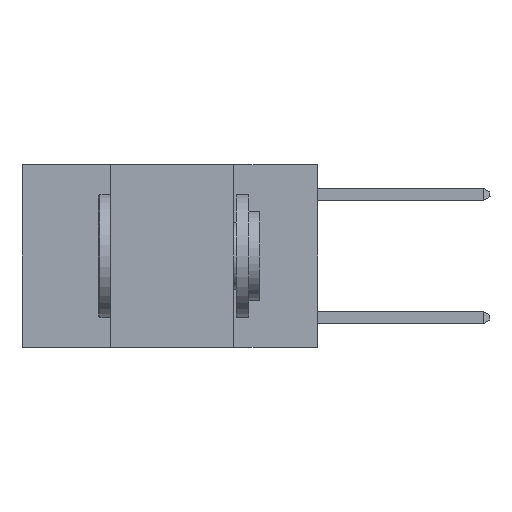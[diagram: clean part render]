
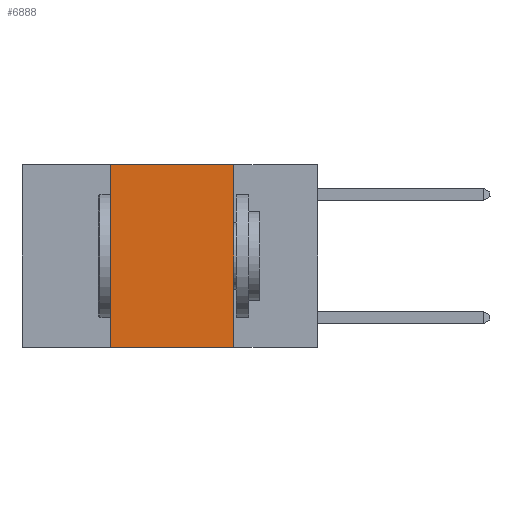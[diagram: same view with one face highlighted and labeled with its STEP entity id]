
A CAD part, left-side view. The second image highlights one B-rep face of the part: STEP entity #6888.
In plain terms, the highlighted planar face has unit normal (-1, 0, 0).
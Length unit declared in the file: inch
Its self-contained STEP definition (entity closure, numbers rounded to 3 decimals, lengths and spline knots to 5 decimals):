
#2115 = DIRECTION ( 'NONE',  ( 0., 0., 1. ) ) ;
#2191 = DIRECTION ( 'NONE',  ( 1., 0., 0. ) ) ;
#2390 = VERTEX_POINT ( 'NONE', #15531 ) ;
#2639 = VECTOR ( 'NONE', #3451, 39.37008 ) ;
#2764 = VECTOR ( 'NONE', #2115, 39.37008 ) ;
#2792 = ORIENTED_EDGE ( 'NONE', *, *, #17667, .F. ) ;
#3072 = CARTESIAN_POINT ( 'NONE',  ( 0., 0.6, 0. ) ) ;
#3198 = EDGE_CURVE ( 'NONE', #15660, #10734, #3631, .T. ) ;
#3207 = VECTOR ( 'NONE', #6868, 39.37008 ) ;
#3451 = DIRECTION ( 'NONE',  ( 0., -1., 0. ) ) ;
#3631 = LINE ( 'NONE', #4788, #10253 ) ;
#4340 = VERTEX_POINT ( 'NONE', #17554 ) ;
#4788 = CARTESIAN_POINT ( 'NONE',  ( 0., 0.17, 0. ) ) ;
#4964 = CARTESIAN_POINT ( 'NONE',  ( 0., 0.6, -0.37 ) ) ;
#6868 = DIRECTION ( 'NONE',  ( 0., -1., 0. ) ) ;
#6888 = ADVANCED_FACE ( 'NONE', ( #14616 ), #8845, .F. ) ;
#7405 = CARTESIAN_POINT ( 'NONE',  ( 0., 0.17, -0.37 ) ) ;
#8462 = LINE ( 'NONE', #3072, #3207 ) ;
#8845 = PLANE ( 'NONE',  #12199 ) ;
#9971 = ORIENTED_EDGE ( 'NONE', *, *, #10574, .T. ) ;
#10092 = CARTESIAN_POINT ( 'NONE',  ( 0., 0.17, 0. ) ) ;
#10253 = VECTOR ( 'NONE', #10283, 39.37008 ) ;
#10283 = DIRECTION ( 'NONE',  ( 0., 0., -1. ) ) ;
#10361 = LINE ( 'NONE', #4964, #2639 ) ;
#10558 = LINE ( 'NONE', #11906, #2764 ) ;
#10574 = EDGE_CURVE ( 'NONE', #2390, #10734, #10361, .T. ) ;
#10734 = VERTEX_POINT ( 'NONE', #7405 ) ;
#11015 = EDGE_CURVE ( 'NONE', #4340, #15660, #8462, .T. ) ;
#11906 = CARTESIAN_POINT ( 'NONE',  ( 0., 0.42, 0. ) ) ;
#12199 = AXIS2_PLACEMENT_3D ( 'NONE', #17311, #2191, #15807 ) ;
#12343 = ORIENTED_EDGE ( 'NONE', *, *, #3198, .F. ) ;
#13605 = EDGE_LOOP ( 'NONE', ( #12343, #15535, #2792, #9971 ) ) ;
#14616 = FACE_OUTER_BOUND ( 'NONE', #13605, .T. ) ;
#15531 = CARTESIAN_POINT ( 'NONE',  ( 0., 0.42, -0.37 ) ) ;
#15535 = ORIENTED_EDGE ( 'NONE', *, *, #11015, .F. ) ;
#15660 = VERTEX_POINT ( 'NONE', #10092 ) ;
#15807 = DIRECTION ( 'NONE',  ( 0., 0., -1. ) ) ;
#17311 = CARTESIAN_POINT ( 'NONE',  ( 0., 0.6, 0. ) ) ;
#17554 = CARTESIAN_POINT ( 'NONE',  ( 0., 0.42, 0. ) ) ;
#17667 = EDGE_CURVE ( 'NONE', #2390, #4340, #10558, .T. ) ;
